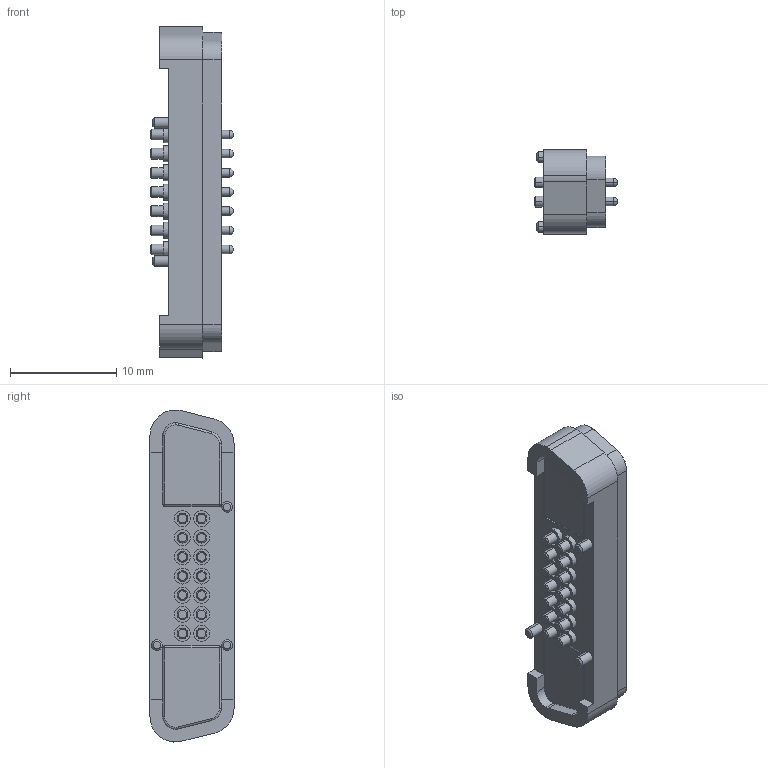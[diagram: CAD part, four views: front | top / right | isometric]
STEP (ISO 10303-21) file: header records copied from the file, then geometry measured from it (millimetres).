
FILE_DESCRIPTION (( 'STEP AP203' ), '1' );
FILE_NAME ('685B1422261115E.STEP', '2023-03-02T12:42:10', ( 'Magnum' ), ( '' ), 'SwSTEP 2.0', 'SolidWorks 2020', '' );
FILE_SCHEMA (( 'CONFIG_CONTROL_DESIGN' ));
Length unit declared in the file: millimetre
Products named in the file (1): 685B1422261115E
Bounding box: 7.8 x 7.9 x 31.2 mm (x, y, z)
Volume: 1155.9 mm3; surface area: 1034.2 mm2
Topology: 1 solids, 1 shells, 341 faces, 772 edges, 463 vertices
Faces by surface type: cylinder 155, plane 82, torus 38, cone 34, sphere 32
Entity records: 9234 total; most frequent: DIRECTION 1813, CARTESIAN_POINT 1520, ORIENTED_EDGE 1424, AXIS2_PLACEMENT_3D 764, EDGE_CURVE 712, VERTEX_POINT 435, CIRCLE 422, EDGE_LOOP 403
